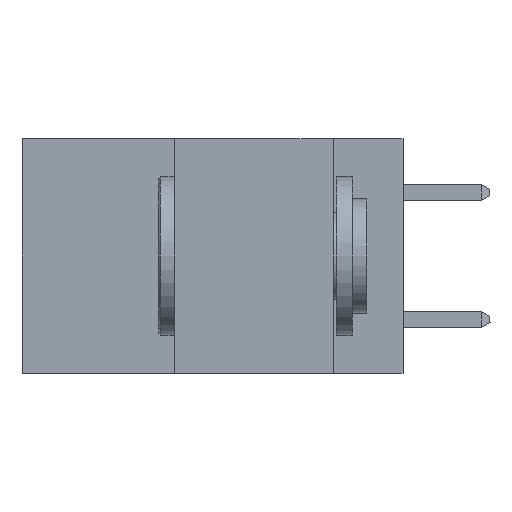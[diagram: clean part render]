
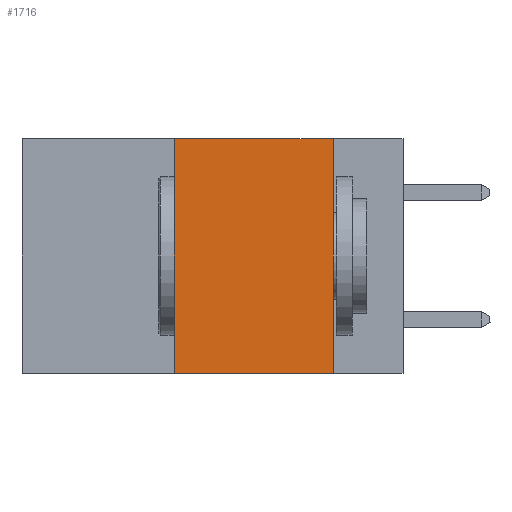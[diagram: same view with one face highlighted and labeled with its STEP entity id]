
A CAD part, left-side view. The second image highlights one B-rep face of the part: STEP entity #1716.
In plain terms, the highlighted planar face has unit normal (-1, 0, 0).
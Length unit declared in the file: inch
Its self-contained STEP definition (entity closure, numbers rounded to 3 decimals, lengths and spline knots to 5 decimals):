
#567 = VERTEX_POINT ( 'NONE', #7948 ) ;
#1716 = ADVANCED_FACE ( 'NONE', ( #11485 ), #18001, .F. ) ;
#1757 = AXIS2_PLACEMENT_3D ( 'NONE', #9846, #17793, #17769 ) ;
#3683 = EDGE_CURVE ( 'NONE', #567, #5854, #13360, .T. ) ;
#4958 = DIRECTION ( 'NONE',  ( 0., -1., 0. ) ) ;
#5280 = CARTESIAN_POINT ( 'NONE',  ( 0., 0.6, 0. ) ) ;
#5281 = ORIENTED_EDGE ( 'NONE', *, *, #17959, .F. ) ;
#5600 = LINE ( 'NONE', #12909, #13402 ) ;
#5818 = VECTOR ( 'NONE', #8334, 39.37008 ) ;
#5854 = VERTEX_POINT ( 'NONE', #9779 ) ;
#5988 = VECTOR ( 'NONE', #17287, 39.37008 ) ;
#6010 = DIRECTION ( 'NONE',  ( 0., 0., 1. ) ) ;
#6241 = EDGE_CURVE ( 'NONE', #9581, #567, #14262, .T. ) ;
#6937 = CARTESIAN_POINT ( 'NONE',  ( 0., 0.6, -0.37 ) ) ;
#7948 = CARTESIAN_POINT ( 'NONE',  ( 0., 0.11, 0. ) ) ;
#8334 = DIRECTION ( 'NONE',  ( 0., -1., 0. ) ) ;
#9581 = VERTEX_POINT ( 'NONE', #11309 ) ;
#9779 = CARTESIAN_POINT ( 'NONE',  ( 0., 0.11, -0.37 ) ) ;
#9846 = CARTESIAN_POINT ( 'NONE',  ( 0., 0.6, 0. ) ) ;
#10603 = VECTOR ( 'NONE', #4958, 39.37008 ) ;
#11309 = CARTESIAN_POINT ( 'NONE',  ( 0., 0.36, 0. ) ) ;
#11485 = FACE_OUTER_BOUND ( 'NONE', #16899, .T. ) ;
#11785 = ORIENTED_EDGE ( 'NONE', *, *, #3683, .F. ) ;
#12020 = VERTEX_POINT ( 'NONE', #12546 ) ;
#12546 = CARTESIAN_POINT ( 'NONE',  ( 0., 0.36, -0.37 ) ) ;
#12909 = CARTESIAN_POINT ( 'NONE',  ( 0., 0.36, 0. ) ) ;
#13360 = LINE ( 'NONE', #17318, #5988 ) ;
#13402 = VECTOR ( 'NONE', #6010, 39.37008 ) ;
#14262 = LINE ( 'NONE', #5280, #10603 ) ;
#15919 = ORIENTED_EDGE ( 'NONE', *, *, #6241, .F. ) ;
#16769 = ORIENTED_EDGE ( 'NONE', *, *, #17099, .T. ) ;
#16879 = LINE ( 'NONE', #6937, #5818 ) ;
#16899 = EDGE_LOOP ( 'NONE', ( #11785, #15919, #5281, #16769 ) ) ;
#17099 = EDGE_CURVE ( 'NONE', #12020, #5854, #16879, .T. ) ;
#17287 = DIRECTION ( 'NONE',  ( 0., 0., -1. ) ) ;
#17318 = CARTESIAN_POINT ( 'NONE',  ( 0., 0.11, 0. ) ) ;
#17769 = DIRECTION ( 'NONE',  ( 0., 0., -1. ) ) ;
#17793 = DIRECTION ( 'NONE',  ( 1., 0., 0. ) ) ;
#17959 = EDGE_CURVE ( 'NONE', #12020, #9581, #5600, .T. ) ;
#18001 = PLANE ( 'NONE',  #1757 ) ;
